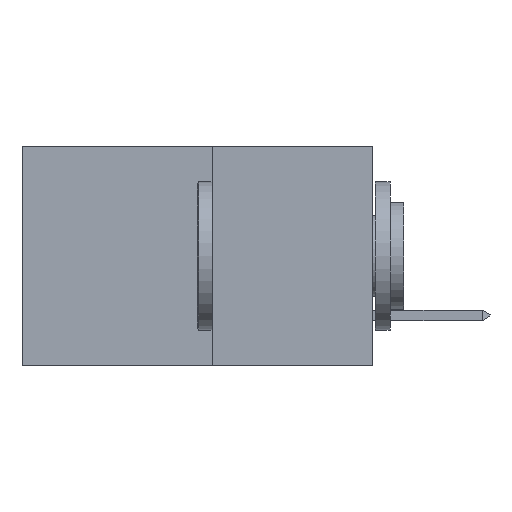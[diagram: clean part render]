
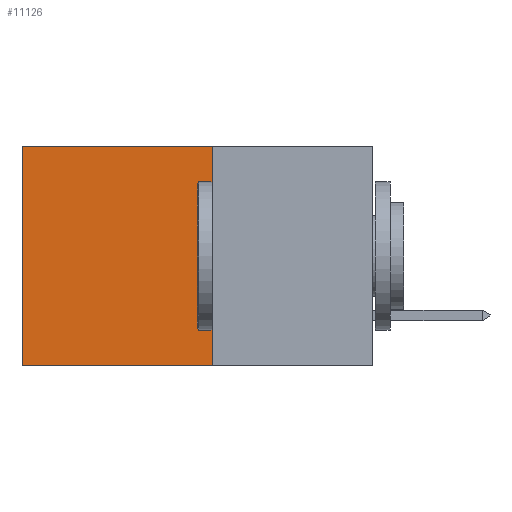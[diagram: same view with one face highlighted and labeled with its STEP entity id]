
A CAD part, left-side view. The second image highlights one B-rep face of the part: STEP entity #11126.
In plain terms, the highlighted planar face has unit normal (-1, 0, 0).
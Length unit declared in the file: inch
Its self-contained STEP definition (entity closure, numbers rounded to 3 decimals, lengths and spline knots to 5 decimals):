
#271 = LINE ( 'NONE', #10935, #5855 ) ;
#559 = CARTESIAN_POINT ( 'NONE',  ( 0.277, 0.27, -0.37 ) ) ;
#1637 = VECTOR ( 'NONE', #7793, 39.37008 ) ;
#1979 = ORIENTED_EDGE ( 'NONE', *, *, #6274, .T. ) ;
#2194 = VECTOR ( 'NONE', #6693, 39.37008 ) ;
#2497 = EDGE_CURVE ( 'NONE', #6596, #8332, #10352, .T. ) ;
#3521 = CARTESIAN_POINT ( 'NONE',  ( 0.277, 0.59, -0.37 ) ) ;
#4039 = CARTESIAN_POINT ( 'NONE',  ( 0.277, 0.59, 0. ) ) ;
#4519 = PLANE ( 'NONE',  #10880 ) ;
#4613 = EDGE_CURVE ( 'NONE', #11497, #8332, #271, .T. ) ;
#5432 = FACE_OUTER_BOUND ( 'NONE', #6427, .T. ) ;
#5632 = EDGE_CURVE ( 'NONE', #6396, #6596, #10259, .T. ) ;
#5660 = DIRECTION ( 'NONE',  ( 1., 0., 0. ) ) ;
#5855 = VECTOR ( 'NONE', #10954, 39.37008 ) ;
#6274 = EDGE_CURVE ( 'NONE', #6396, #11497, #13312, .T. ) ;
#6396 = VERTEX_POINT ( 'NONE', #10155 ) ;
#6427 = EDGE_LOOP ( 'NONE', ( #8045, #6671, #11947, #1979 ) ) ;
#6596 = VERTEX_POINT ( 'NONE', #559 ) ;
#6671 = ORIENTED_EDGE ( 'NONE', *, *, #2497, .F. ) ;
#6693 = DIRECTION ( 'NONE',  ( 0., 0., -1. ) ) ;
#6726 = CARTESIAN_POINT ( 'NONE',  ( 0.277, 0.27, -0.37 ) ) ;
#7793 = DIRECTION ( 'NONE',  ( 0., 1., 0. ) ) ;
#7810 = VECTOR ( 'NONE', #8982, 39.37008 ) ;
#8045 = ORIENTED_EDGE ( 'NONE', *, *, #4613, .T. ) ;
#8332 = VERTEX_POINT ( 'NONE', #3521 ) ;
#8982 = DIRECTION ( 'NONE',  ( 0., 1., 0. ) ) ;
#9883 = CARTESIAN_POINT ( 'NONE',  ( 0.277, 0.27, -0.37 ) ) ;
#10155 = CARTESIAN_POINT ( 'NONE',  ( 0.277, 0.27, 0. ) ) ;
#10259 = LINE ( 'NONE', #6726, #2194 ) ;
#10352 = LINE ( 'NONE', #9883, #7810 ) ;
#10880 = AXIS2_PLACEMENT_3D ( 'NONE', #11100, #5660, #13294 ) ;
#10935 = CARTESIAN_POINT ( 'NONE',  ( 0.277, 0.59, -0.37 ) ) ;
#10954 = DIRECTION ( 'NONE',  ( 0., 0., -1. ) ) ;
#11100 = CARTESIAN_POINT ( 'NONE',  ( 0.277, 0.27, -0.37 ) ) ;
#11126 = ADVANCED_FACE ( 'NONE', ( #5432 ), #4519, .F. ) ;
#11497 = VERTEX_POINT ( 'NONE', #4039 ) ;
#11947 = ORIENTED_EDGE ( 'NONE', *, *, #5632, .F. ) ;
#13214 = CARTESIAN_POINT ( 'NONE',  ( 0.277, 0.27, 0. ) ) ;
#13294 = DIRECTION ( 'NONE',  ( 0., 0., -1. ) ) ;
#13312 = LINE ( 'NONE', #13214, #1637 ) ;
